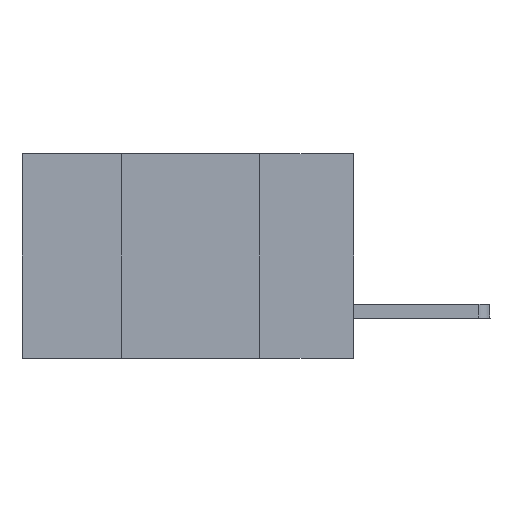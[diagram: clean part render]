
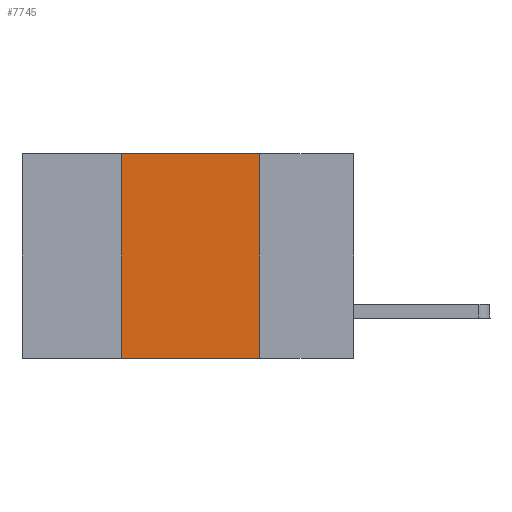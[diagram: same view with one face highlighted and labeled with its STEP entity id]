
A CAD part, left-side view. The second image highlights one B-rep face of the part: STEP entity #7745.
In plain terms, the highlighted planar face has unit normal (-1, 0, 0).
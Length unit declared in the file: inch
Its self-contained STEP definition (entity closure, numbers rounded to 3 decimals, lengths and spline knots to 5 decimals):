
#629 = DIRECTION ( 'NONE',  ( 0., -1., 0. ) ) ;
#1172 = VERTEX_POINT ( 'NONE', #13214 ) ;
#1782 = CARTESIAN_POINT ( 'NONE',  ( 0., 0.17, 0. ) ) ;
#1821 = ORIENTED_EDGE ( 'NONE', *, *, #13272, .F. ) ;
#2028 = LINE ( 'NONE', #10234, #12973 ) ;
#2141 = ORIENTED_EDGE ( 'NONE', *, *, #7070, .F. ) ;
#2796 = CARTESIAN_POINT ( 'NONE',  ( 0., 0.6, -0.37 ) ) ;
#3092 = CARTESIAN_POINT ( 'NONE',  ( 0., 0.42, 0. ) ) ;
#3398 = VERTEX_POINT ( 'NONE', #1782 ) ;
#3487 = VERTEX_POINT ( 'NONE', #3092 ) ;
#3736 = EDGE_CURVE ( 'NONE', #10813, #1172, #12956, .T. ) ;
#3846 = EDGE_CURVE ( 'NONE', #10813, #3487, #9974, .T. ) ;
#4925 = DIRECTION ( 'NONE',  ( 0., 0., -1. ) ) ;
#5103 = PLANE ( 'NONE',  #9132 ) ;
#5536 = DIRECTION ( 'NONE',  ( 0., 0., 1. ) ) ;
#6374 = LINE ( 'NONE', #8522, #8040 ) ;
#7070 = EDGE_CURVE ( 'NONE', #3398, #1172, #2028, .T. ) ;
#7147 = DIRECTION ( 'NONE',  ( 0., 0., -1. ) ) ;
#7459 = EDGE_LOOP ( 'NONE', ( #2141, #1821, #12182, #9895 ) ) ;
#7618 = FACE_OUTER_BOUND ( 'NONE', #7459, .T. ) ;
#7745 = ADVANCED_FACE ( 'NONE', ( #7618 ), #5103, .F. ) ;
#8040 = VECTOR ( 'NONE', #12750, 39.37008 ) ;
#8522 = CARTESIAN_POINT ( 'NONE',  ( 0., 0.6, 0. ) ) ;
#9132 = AXIS2_PLACEMENT_3D ( 'NONE', #13615, #11285, #4925 ) ;
#9895 = ORIENTED_EDGE ( 'NONE', *, *, #3736, .T. ) ;
#9974 = LINE ( 'NONE', #13100, #12803 ) ;
#10234 = CARTESIAN_POINT ( 'NONE',  ( 0., 0.17, 0. ) ) ;
#10813 = VERTEX_POINT ( 'NONE', #10925 ) ;
#10925 = CARTESIAN_POINT ( 'NONE',  ( 0., 0.42, -0.37 ) ) ;
#11285 = DIRECTION ( 'NONE',  ( 1., 0., 0. ) ) ;
#12182 = ORIENTED_EDGE ( 'NONE', *, *, #3846, .F. ) ;
#12292 = VECTOR ( 'NONE', #629, 39.37008 ) ;
#12750 = DIRECTION ( 'NONE',  ( 0., -1., 0. ) ) ;
#12803 = VECTOR ( 'NONE', #5536, 39.37008 ) ;
#12956 = LINE ( 'NONE', #2796, #12292 ) ;
#12973 = VECTOR ( 'NONE', #7147, 39.37008 ) ;
#13100 = CARTESIAN_POINT ( 'NONE',  ( 0., 0.42, 0. ) ) ;
#13214 = CARTESIAN_POINT ( 'NONE',  ( 0., 0.17, -0.37 ) ) ;
#13272 = EDGE_CURVE ( 'NONE', #3487, #3398, #6374, .T. ) ;
#13615 = CARTESIAN_POINT ( 'NONE',  ( 0., 0.6, 0. ) ) ;
